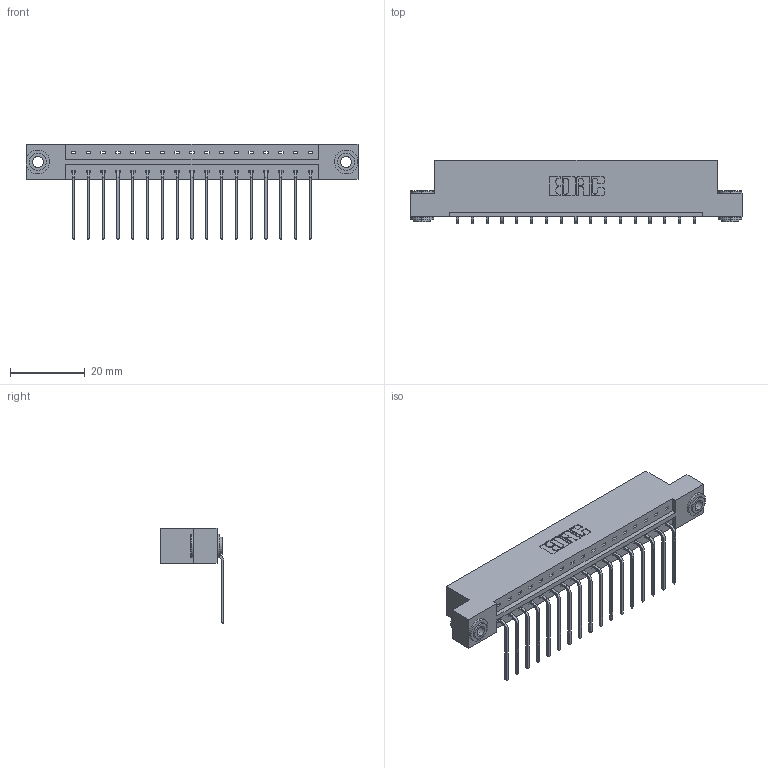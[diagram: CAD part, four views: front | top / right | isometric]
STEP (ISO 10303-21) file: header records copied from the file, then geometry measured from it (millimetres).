
FILE_DESCRIPTION (( 'STEP AP203' ), '1' );
FILE_NAME ('833-017-559-103.STEP', '2020-05-31T20:36:44', ( '' ), ( '' ), 'SwSTEP 2.0', 'SolidWorks 2020', '' );
FILE_SCHEMA (( 'CONFIG_CONTROL_DESIGN' ));
Length unit declared in the file: inch
Products named in the file (4): 345-292-001_558 559 Tail - 1; 833-017-559-103; 345-250-002_345-250-002-102; 833 Part_Flush - .156 Dia - TH
Assembly tree (20 placements, depth 2):
  833-017-559-103
    833 Part_Flush - .156 Dia - TH
    345-292-001_558 559 Tail - 1  x17
    345-250-002_345-250-002-102  x2
Bounding box: 88.9 x 17.09 x 25.53 mm (x, y, z)
Volume: 8806.9 mm3; surface area: 9940.1 mm2
Topology: 20 solids, 20 shells, 1172 faces, 3481 edges, 2294 vertices
Faces by surface type: plane 828, cylinder 336, cone 8
Entity records: 14360 total; most frequent: CARTESIAN_POINT 2460, ORIENTED_EDGE 2406, DIRECTION 2159, EDGE_CURVE 1203, VECTOR 1051, LINE 1051, VERTEX_POINT 798, AXIS2_PLACEMENT_3D 554
